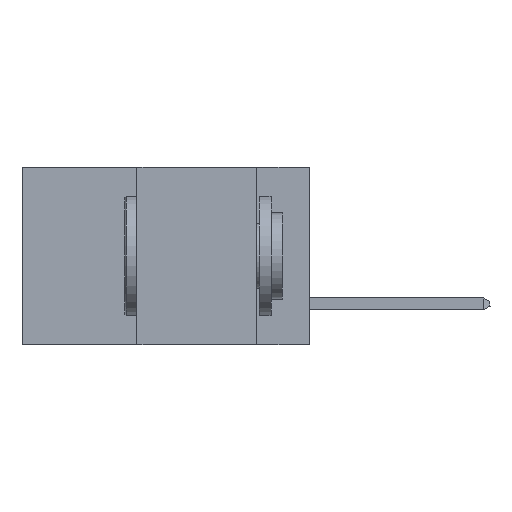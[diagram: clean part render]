
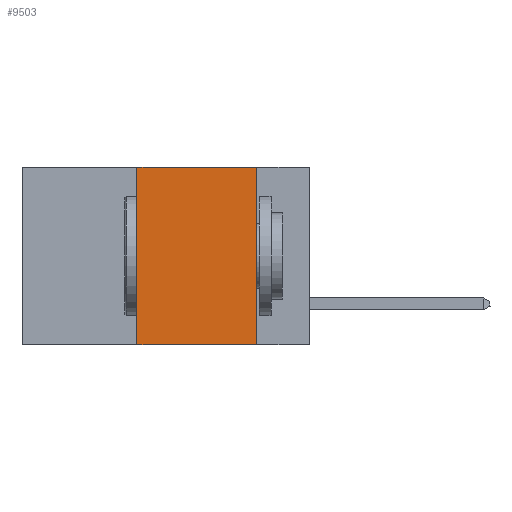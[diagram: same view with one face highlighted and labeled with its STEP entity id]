
A CAD part, left-side view. The second image highlights one B-rep face of the part: STEP entity #9503.
In plain terms, the highlighted planar face has unit normal (-1, 0, 0).
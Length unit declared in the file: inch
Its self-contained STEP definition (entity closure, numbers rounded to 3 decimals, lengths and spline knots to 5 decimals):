
#68 = EDGE_LOOP ( 'NONE', ( #17622, #17762, #13431, #1779 ) ) ;
#130 = VERTEX_POINT ( 'NONE', #16675 ) ;
#182 = PLANE ( 'NONE',  #9337 ) ;
#667 = LINE ( 'NONE', #2987, #11655 ) ;
#1717 = CARTESIAN_POINT ( 'NONE',  ( 0., 0.36, 0. ) ) ;
#1749 = CARTESIAN_POINT ( 'NONE',  ( 0., 0.6, -0.37 ) ) ;
#1779 = ORIENTED_EDGE ( 'NONE', *, *, #4323, .T. ) ;
#2556 = VERTEX_POINT ( 'NONE', #1717 ) ;
#2987 = CARTESIAN_POINT ( 'NONE',  ( 0., 0.6, 0. ) ) ;
#3103 = DIRECTION ( 'NONE',  ( 0., -1., 0. ) ) ;
#3915 = LINE ( 'NONE', #1749, #18001 ) ;
#4023 = EDGE_CURVE ( 'NONE', #2556, #15688, #667, .T. ) ;
#4323 = EDGE_CURVE ( 'NONE', #11714, #130, #3915, .T. ) ;
#5169 = VECTOR ( 'NONE', #8483, 39.37008 ) ;
#5275 = DIRECTION ( 'NONE',  ( 1., 0., 0. ) ) ;
#5424 = EDGE_CURVE ( 'NONE', #11714, #2556, #8479, .T. ) ;
#6344 = LINE ( 'NONE', #17641, #17361 ) ;
#8479 = LINE ( 'NONE', #16911, #5169 ) ;
#8483 = DIRECTION ( 'NONE',  ( 0., 0., 1. ) ) ;
#9337 = AXIS2_PLACEMENT_3D ( 'NONE', #11119, #5275, #13692 ) ;
#9503 = ADVANCED_FACE ( 'NONE', ( #12708 ), #182, .F. ) ;
#10418 = DIRECTION ( 'NONE',  ( 0., -1., 0. ) ) ;
#10613 = CARTESIAN_POINT ( 'NONE',  ( 0., 0.36, -0.37 ) ) ;
#11119 = CARTESIAN_POINT ( 'NONE',  ( 0., 0.6, 0. ) ) ;
#11655 = VECTOR ( 'NONE', #3103, 39.37008 ) ;
#11714 = VERTEX_POINT ( 'NONE', #10613 ) ;
#12708 = FACE_OUTER_BOUND ( 'NONE', #68, .T. ) ;
#13431 = ORIENTED_EDGE ( 'NONE', *, *, #5424, .F. ) ;
#13692 = DIRECTION ( 'NONE',  ( 0., 0., -1. ) ) ;
#15688 = VERTEX_POINT ( 'NONE', #17618 ) ;
#16054 = DIRECTION ( 'NONE',  ( 0., 0., -1. ) ) ;
#16675 = CARTESIAN_POINT ( 'NONE',  ( 0., 0.11, -0.37 ) ) ;
#16911 = CARTESIAN_POINT ( 'NONE',  ( 0., 0.36, 0. ) ) ;
#17361 = VECTOR ( 'NONE', #16054, 39.37008 ) ;
#17618 = CARTESIAN_POINT ( 'NONE',  ( 0., 0.11, 0. ) ) ;
#17622 = ORIENTED_EDGE ( 'NONE', *, *, #18207, .F. ) ;
#17641 = CARTESIAN_POINT ( 'NONE',  ( 0., 0.11, 0. ) ) ;
#17762 = ORIENTED_EDGE ( 'NONE', *, *, #4023, .F. ) ;
#18001 = VECTOR ( 'NONE', #10418, 39.37008 ) ;
#18207 = EDGE_CURVE ( 'NONE', #15688, #130, #6344, .T. ) ;
